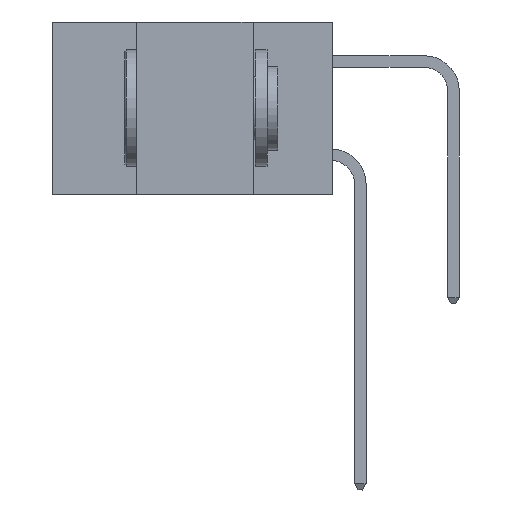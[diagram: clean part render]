
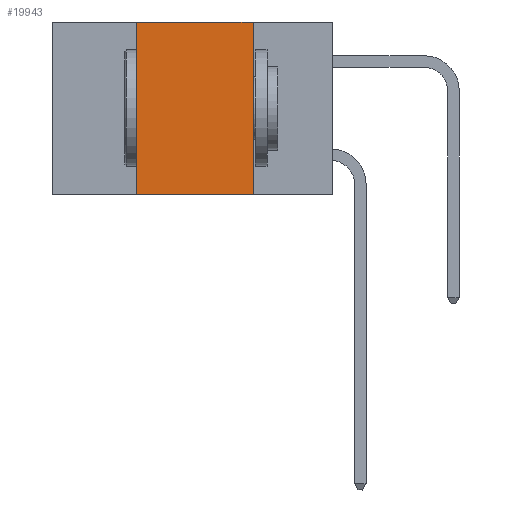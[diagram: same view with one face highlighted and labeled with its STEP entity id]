
A CAD part, left-side view. The second image highlights one B-rep face of the part: STEP entity #19943.
In plain terms, the highlighted planar face has unit normal (-1, 0, 0).
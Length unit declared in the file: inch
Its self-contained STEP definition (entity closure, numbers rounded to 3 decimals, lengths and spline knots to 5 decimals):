
#412 = AXIS2_PLACEMENT_3D ( 'NONE', #8653, #10427, #12434 ) ;
#1073 = CARTESIAN_POINT ( 'NONE',  ( 0., 0.6, 0. ) ) ;
#2486 = EDGE_CURVE ( 'NONE', #8069, #19855, #7702, .T. ) ;
#2714 = DIRECTION ( 'NONE',  ( 0., -1., 0. ) ) ;
#2873 = ORIENTED_EDGE ( 'NONE', *, *, #2486, .F. ) ;
#3002 = VECTOR ( 'NONE', #6921, 39.37008 ) ;
#3749 = PLANE ( 'NONE',  #412 ) ;
#3759 = ORIENTED_EDGE ( 'NONE', *, *, #9820, .F. ) ;
#3860 = CARTESIAN_POINT ( 'NONE',  ( 0., 0.17, 0. ) ) ;
#4160 = VECTOR ( 'NONE', #20485, 39.37008 ) ;
#6412 = LINE ( 'NONE', #13419, #9255 ) ;
#6812 = CARTESIAN_POINT ( 'NONE',  ( 0., 0.42, -0.37 ) ) ;
#6921 = DIRECTION ( 'NONE',  ( 0., -1., 0. ) ) ;
#7405 = CARTESIAN_POINT ( 'NONE',  ( 0., 0.42, 0. ) ) ;
#7702 = LINE ( 'NONE', #1073, #13780 ) ;
#8069 = VERTEX_POINT ( 'NONE', #7405 ) ;
#8098 = ORIENTED_EDGE ( 'NONE', *, *, #13188, .F. ) ;
#8357 = EDGE_CURVE ( 'NONE', #18424, #8722, #15289, .T. ) ;
#8653 = CARTESIAN_POINT ( 'NONE',  ( 0., 0.6, 0. ) ) ;
#8722 = VERTEX_POINT ( 'NONE', #18810 ) ;
#9255 = VECTOR ( 'NONE', #19967, 39.37008 ) ;
#9820 = EDGE_CURVE ( 'NONE', #19855, #8722, #6412, .T. ) ;
#10427 = DIRECTION ( 'NONE',  ( 1., 0., 0. ) ) ;
#12434 = DIRECTION ( 'NONE',  ( 0., 0., -1. ) ) ;
#13188 = EDGE_CURVE ( 'NONE', #18424, #8069, #18826, .T. ) ;
#13419 = CARTESIAN_POINT ( 'NONE',  ( 0., 0.17, -0.37 ) ) ;
#13780 = VECTOR ( 'NONE', #2714, 39.37008 ) ;
#13841 = CARTESIAN_POINT ( 'NONE',  ( 0., 0.6, -0.37 ) ) ;
#14054 = CARTESIAN_POINT ( 'NONE',  ( 0., 0.42, -0.37 ) ) ;
#15289 = LINE ( 'NONE', #13841, #3002 ) ;
#16958 = EDGE_LOOP ( 'NONE', ( #3759, #2873, #8098, #20367 ) ) ;
#18424 = VERTEX_POINT ( 'NONE', #14054 ) ;
#18810 = CARTESIAN_POINT ( 'NONE',  ( 0., 0.17, -0.37 ) ) ;
#18826 = LINE ( 'NONE', #6812, #4160 ) ;
#19855 = VERTEX_POINT ( 'NONE', #3860 ) ;
#19943 = ADVANCED_FACE ( 'NONE', ( #20857 ), #3749, .F. ) ;
#19967 = DIRECTION ( 'NONE',  ( 0., 0., -1. ) ) ;
#20367 = ORIENTED_EDGE ( 'NONE', *, *, #8357, .T. ) ;
#20485 = DIRECTION ( 'NONE',  ( 0., 0., 1. ) ) ;
#20857 = FACE_OUTER_BOUND ( 'NONE', #16958, .T. ) ;
